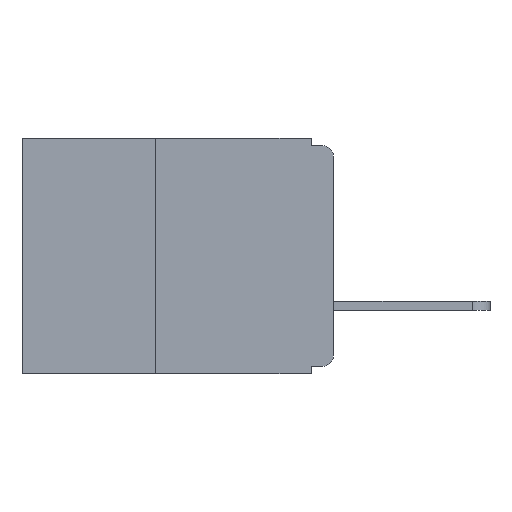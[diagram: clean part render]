
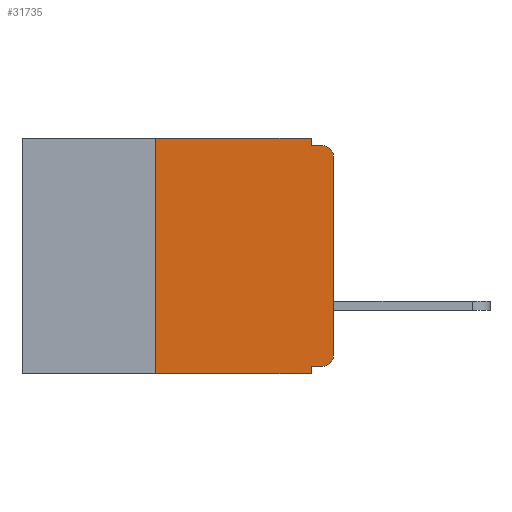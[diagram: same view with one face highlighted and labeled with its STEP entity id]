
A CAD part, left-side view. The second image highlights one B-rep face of the part: STEP entity #31735.
In plain terms, the highlighted planar face has unit normal (-1, 0, 0).
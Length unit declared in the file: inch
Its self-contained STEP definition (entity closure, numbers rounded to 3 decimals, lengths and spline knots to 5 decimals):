
#343 = ORIENTED_EDGE ( 'NONE', *, *, #7518, .T. ) ;
#820 = VECTOR ( 'NONE', #4756, 39.37008 ) ;
#930 = ORIENTED_EDGE ( 'NONE', *, *, #21041, .F. ) ;
#1420 = CARTESIAN_POINT ( 'NONE',  ( 0., 0., -0.025 ) ) ;
#2318 = VECTOR ( 'NONE', #7633, 39.37008 ) ;
#3254 = CARTESIAN_POINT ( 'NONE',  ( 0., 0.437, 0. ) ) ;
#3707 = CARTESIAN_POINT ( 'NONE',  ( 0., 0.031, -0.01 ) ) ;
#4756 = DIRECTION ( 'NONE',  ( 0., 1., 0. ) ) ;
#4783 = PLANE ( 'NONE',  #12148 ) ;
#5121 = VECTOR ( 'NONE', #12908, 39.37008 ) ;
#5857 = DIRECTION ( 'NONE',  ( 0., -1., 0. ) ) ;
#5895 = CARTESIAN_POINT ( 'NONE',  ( 0., 0.031, 0. ) ) ;
#5934 = EDGE_CURVE ( 'NONE', #24849, #27845, #15944, .T. ) ;
#5983 = CARTESIAN_POINT ( 'NONE',  ( 0., 0.031, -0.33 ) ) ;
#6003 = DIRECTION ( 'NONE',  ( 0., -1., 0. ) ) ;
#6344 = CARTESIAN_POINT ( 'NONE',  ( 0., 0.031, -0.32 ) ) ;
#6674 = DIRECTION ( 'NONE',  ( 0., 0., -1. ) ) ;
#6745 = CARTESIAN_POINT ( 'NONE',  ( 0., 0.031, -0.33 ) ) ;
#7518 = EDGE_CURVE ( 'NONE', #27845, #30268, #20592, .T. ) ;
#7633 = DIRECTION ( 'NONE',  ( 0., 0., 1. ) ) ;
#7838 = CARTESIAN_POINT ( 'NONE',  ( 0., 0., 0. ) ) ;
#8277 = EDGE_CURVE ( 'NONE', #22058, #24849, #25204, .T. ) ;
#8523 = LINE ( 'NONE', #12627, #820 ) ;
#8844 = ORIENTED_EDGE ( 'NONE', *, *, #27079, .F. ) ;
#8997 = EDGE_CURVE ( 'NONE', #18844, #9026, #29788, .T. ) ;
#9026 = VERTEX_POINT ( 'NONE', #5983 ) ;
#10004 = DIRECTION ( 'NONE',  ( 1., 0., 0. ) ) ;
#11405 = DIRECTION ( 'NONE',  ( 0., 0., -1. ) ) ;
#12054 = ORIENTED_EDGE ( 'NONE', *, *, #23561, .T. ) ;
#12148 = AXIS2_PLACEMENT_3D ( 'NONE', #25075, #10004, #27569 ) ;
#12627 = CARTESIAN_POINT ( 'NONE',  ( 0., 0., -0.32 ) ) ;
#12908 = DIRECTION ( 'NONE',  ( 0., 0., 1. ) ) ;
#14391 = ORIENTED_EDGE ( 'NONE', *, *, #28868, .F. ) ;
#14743 = ORIENTED_EDGE ( 'NONE', *, *, #5934, .T. ) ;
#15523 = CARTESIAN_POINT ( 'NONE',  ( 0., 0., -0.305 ) ) ;
#15685 = LINE ( 'NONE', #31440, #17280 ) ;
#15776 = AXIS2_PLACEMENT_3D ( 'NONE', #30661, #30628, #30598 ) ;
#15944 = LINE ( 'NONE', #7838, #2318 ) ;
#17280 = VECTOR ( 'NONE', #11405, 39.37008 ) ;
#17363 = EDGE_LOOP ( 'NONE', ( #14743, #343, #8844, #14391, #21137, #23098, #12054, #31651, #930, #28685 ) ) ;
#18844 = VERTEX_POINT ( 'NONE', #6344 ) ;
#19168 = DIRECTION ( 'NONE',  ( 0., 0., -1. ) ) ;
#19172 = DIRECTION ( 'NONE',  ( -1., 0., 0. ) ) ;
#19232 = CARTESIAN_POINT ( 'NONE',  ( 0., 0.015, -0.305 ) ) ;
#20436 = VECTOR ( 'NONE', #6003, 39.37008 ) ;
#20592 = CIRCLE ( 'NONE', #15776, 0.015 ) ;
#21041 = EDGE_CURVE ( 'NONE', #22058, #18844, #8523, .T. ) ;
#21129 = LINE ( 'NONE', #3254, #32758 ) ;
#21137 = ORIENTED_EDGE ( 'NONE', *, *, #21895, .F. ) ;
#21292 = FACE_OUTER_BOUND ( 'NONE', #17363, .T. ) ;
#21329 = VERTEX_POINT ( 'NONE', #5895 ) ;
#21739 = CARTESIAN_POINT ( 'NONE',  ( 0., 0.015, -0.32 ) ) ;
#21895 = EDGE_CURVE ( 'NONE', #32544, #21329, #21129, .T. ) ;
#22058 = VERTEX_POINT ( 'NONE', #21739 ) ;
#23098 = ORIENTED_EDGE ( 'NONE', *, *, #31217, .F. ) ;
#23299 = CARTESIAN_POINT ( 'NONE',  ( 0., 0.015, -0.01 ) ) ;
#23561 = EDGE_CURVE ( 'NONE', #25685, #9026, #26148, .T. ) ;
#23750 = CARTESIAN_POINT ( 'NONE',  ( 0., 0., -0.01 ) ) ;
#24485 = CARTESIAN_POINT ( 'NONE',  ( 0., 0.25, -0.33 ) ) ;
#24702 = CARTESIAN_POINT ( 'NONE',  ( 0., 0.25, 0. ) ) ;
#24849 = VERTEX_POINT ( 'NONE', #15523 ) ;
#25075 = CARTESIAN_POINT ( 'NONE',  ( 0., 0.437, 0. ) ) ;
#25204 = CIRCLE ( 'NONE', #27948, 0.015 ) ;
#25366 = VECTOR ( 'NONE', #30538, 39.37008 ) ;
#25549 = CARTESIAN_POINT ( 'NONE',  ( 0., 0.437, -0.33 ) ) ;
#25685 = VERTEX_POINT ( 'NONE', #24485 ) ;
#26148 = LINE ( 'NONE', #25549, #25366 ) ;
#26173 = VERTEX_POINT ( 'NONE', #3707 ) ;
#27079 = EDGE_CURVE ( 'NONE', #26173, #30268, #27827, .T. ) ;
#27569 = DIRECTION ( 'NONE',  ( 0., 0., -1. ) ) ;
#27827 = LINE ( 'NONE', #23750, #20436 ) ;
#27845 = VERTEX_POINT ( 'NONE', #1420 ) ;
#27927 = CARTESIAN_POINT ( 'NONE',  ( 0., 0.25, -0.33 ) ) ;
#27948 = AXIS2_PLACEMENT_3D ( 'NONE', #19232, #19172, #19168 ) ;
#28267 = VECTOR ( 'NONE', #6674, 39.37008 ) ;
#28685 = ORIENTED_EDGE ( 'NONE', *, *, #8277, .T. ) ;
#28868 = EDGE_CURVE ( 'NONE', #21329, #26173, #15685, .T. ) ;
#29788 = LINE ( 'NONE', #6745, #28267 ) ;
#30268 = VERTEX_POINT ( 'NONE', #23299 ) ;
#30538 = DIRECTION ( 'NONE',  ( 0., -1., 0. ) ) ;
#30598 = DIRECTION ( 'NONE',  ( 0., 0., -1. ) ) ;
#30628 = DIRECTION ( 'NONE',  ( -1., 0., 0. ) ) ;
#30661 = CARTESIAN_POINT ( 'NONE',  ( 0., 0.015, -0.025 ) ) ;
#31172 = LINE ( 'NONE', #27927, #5121 ) ;
#31217 = EDGE_CURVE ( 'NONE', #25685, #32544, #31172, .T. ) ;
#31440 = CARTESIAN_POINT ( 'NONE',  ( 0., 0.031, 0. ) ) ;
#31651 = ORIENTED_EDGE ( 'NONE', *, *, #8997, .F. ) ;
#31735 = ADVANCED_FACE ( 'NONE', ( #21292 ), #4783, .F. ) ;
#32544 = VERTEX_POINT ( 'NONE', #24702 ) ;
#32758 = VECTOR ( 'NONE', #5857, 39.37008 ) ;
